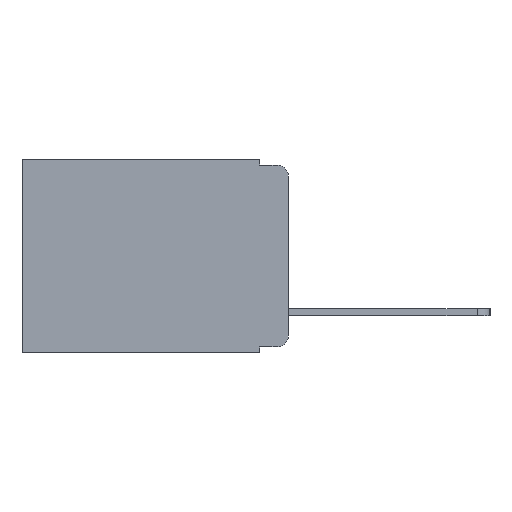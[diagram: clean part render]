
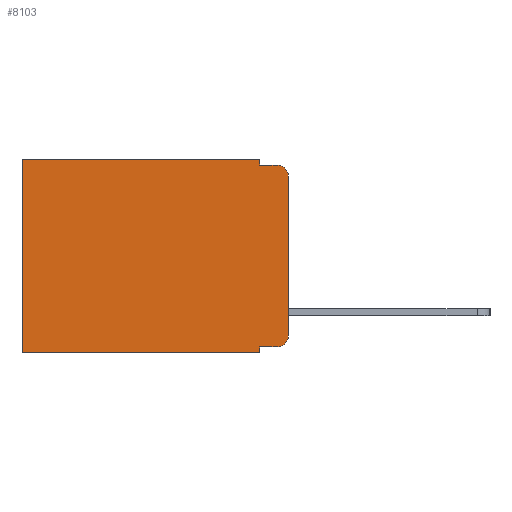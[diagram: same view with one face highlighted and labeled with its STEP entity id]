
A CAD part, left-side view. The second image highlights one B-rep face of the part: STEP entity #8103.
In plain terms, the highlighted planar face has unit normal (-1, 0, 0).
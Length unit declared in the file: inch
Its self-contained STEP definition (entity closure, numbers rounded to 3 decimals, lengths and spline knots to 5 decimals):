
#501 = EDGE_CURVE ( 'NONE', #8266, #10740, #7500, .T. ) ;
#517 = VECTOR ( 'NONE', #9543, 39.37008 ) ;
#1205 = CARTESIAN_POINT ( 'NONE',  ( 0.298, 0., -0.03 ) ) ;
#1229 = LINE ( 'NONE', #2038, #6552 ) ;
#1471 = CARTESIAN_POINT ( 'NONE',  ( 0.298, 0.051, -0.01 ) ) ;
#1753 = CARTESIAN_POINT ( 'NONE',  ( 0.298, 0., -0.313 ) ) ;
#1886 = AXIS2_PLACEMENT_3D ( 'NONE', #12120, #12117, #11517 ) ;
#1944 = EDGE_CURVE ( 'NONE', #9816, #8266, #6136, .T. ) ;
#2038 = CARTESIAN_POINT ( 'NONE',  ( 0.298, 0.473, 0. ) ) ;
#2200 = AXIS2_PLACEMENT_3D ( 'NONE', #4067, #11360, #5139 ) ;
#2552 = CARTESIAN_POINT ( 'NONE',  ( 0.298, 0., 0. ) ) ;
#2587 = ORIENTED_EDGE ( 'NONE', *, *, #13192, .T. ) ;
#2833 = EDGE_CURVE ( 'NONE', #11687, #9010, #9664, .T. ) ;
#2908 = CARTESIAN_POINT ( 'NONE',  ( 0.298, 0.051, 0. ) ) ;
#2997 = EDGE_CURVE ( 'NONE', #3891, #12537, #10493, .T. ) ;
#3063 = ORIENTED_EDGE ( 'NONE', *, *, #11954, .F. ) ;
#3673 = LINE ( 'NONE', #8259, #8922 ) ;
#3827 = ORIENTED_EDGE ( 'NONE', *, *, #2833, .F. ) ;
#3891 = VERTEX_POINT ( 'NONE', #8270 ) ;
#4067 = CARTESIAN_POINT ( 'NONE',  ( 0.298, 0.02, -0.313 ) ) ;
#4087 = VECTOR ( 'NONE', #10235, 39.37008 ) ;
#4259 = CARTESIAN_POINT ( 'NONE',  ( 0.298, 0.02, -0.01 ) ) ;
#4471 = VECTOR ( 'NONE', #4760, 39.37008 ) ;
#4632 = VECTOR ( 'NONE', #11917, 39.37008 ) ;
#4685 = DIRECTION ( 'NONE',  ( 0., 0., -1. ) ) ;
#4690 = ORIENTED_EDGE ( 'NONE', *, *, #12621, .T. ) ;
#4722 = CARTESIAN_POINT ( 'NONE',  ( 0.298, 0.051, -0.01 ) ) ;
#4760 = DIRECTION ( 'NONE',  ( 0., -1., 0. ) ) ;
#4903 = VECTOR ( 'NONE', #12375, 39.37008 ) ;
#5139 = DIRECTION ( 'NONE',  ( 0., 0., -1. ) ) ;
#5840 = VERTEX_POINT ( 'NONE', #1753 ) ;
#5953 = EDGE_CURVE ( 'NONE', #12736, #9010, #7217, .T. ) ;
#6136 = LINE ( 'NONE', #9500, #517 ) ;
#6187 = ORIENTED_EDGE ( 'NONE', *, *, #11328, .F. ) ;
#6552 = VECTOR ( 'NONE', #9326, 39.37008 ) ;
#6600 = DIRECTION ( 'NONE',  ( 0., -1., 0. ) ) ;
#6691 = EDGE_LOOP ( 'NONE', ( #3063, #11713, #3827, #6187, #9414, #4690, #7978, #11766, #10893, #2587 ) ) ;
#6932 = EDGE_CURVE ( 'NONE', #9816, #9827, #3673, .T. ) ;
#7217 = CIRCLE ( 'NONE', #1886, 0.02 ) ;
#7500 = LINE ( 'NONE', #10459, #13256 ) ;
#7978 = ORIENTED_EDGE ( 'NONE', *, *, #501, .F. ) ;
#8103 = ADVANCED_FACE ( 'NONE', ( #12605 ), #9861, .F. ) ;
#8230 = CARTESIAN_POINT ( 'NONE',  ( 0.298, 0.473, -0.343 ) ) ;
#8259 = CARTESIAN_POINT ( 'NONE',  ( 0.298, 0.051, -0.333 ) ) ;
#8266 = VERTEX_POINT ( 'NONE', #9091 ) ;
#8270 = CARTESIAN_POINT ( 'NONE',  ( 0.298, 0.051, 0. ) ) ;
#8785 = CARTESIAN_POINT ( 'NONE',  ( 0.298, 0.02, -0.333 ) ) ;
#8922 = VECTOR ( 'NONE', #6600, 39.37008 ) ;
#9010 = VERTEX_POINT ( 'NONE', #4259 ) ;
#9091 = CARTESIAN_POINT ( 'NONE',  ( 0.298, 0.051, -0.343 ) ) ;
#9188 = CARTESIAN_POINT ( 'NONE',  ( 0.298, 0.473, 0. ) ) ;
#9326 = DIRECTION ( 'NONE',  ( 0., 0., -1. ) ) ;
#9414 = ORIENTED_EDGE ( 'NONE', *, *, #2997, .T. ) ;
#9500 = CARTESIAN_POINT ( 'NONE',  ( 0.298, 0.051, 0. ) ) ;
#9543 = DIRECTION ( 'NONE',  ( 0., 0., -1. ) ) ;
#9664 = LINE ( 'NONE', #4722, #4471 ) ;
#9816 = VERTEX_POINT ( 'NONE', #11867 ) ;
#9827 = VERTEX_POINT ( 'NONE', #8785 ) ;
#9861 = PLANE ( 'NONE',  #9883 ) ;
#9883 = AXIS2_PLACEMENT_3D ( 'NONE', #2552, #10917, #4685 ) ;
#9952 = LINE ( 'NONE', #2908, #4087 ) ;
#10235 = DIRECTION ( 'NONE',  ( 0., 0., -1. ) ) ;
#10459 = CARTESIAN_POINT ( 'NONE',  ( 0.298, 0., -0.343 ) ) ;
#10493 = LINE ( 'NONE', #12842, #4632 ) ;
#10740 = VERTEX_POINT ( 'NONE', #8230 ) ;
#10893 = ORIENTED_EDGE ( 'NONE', *, *, #6932, .T. ) ;
#10917 = DIRECTION ( 'NONE',  ( 1., 0., 0. ) ) ;
#11024 = DIRECTION ( 'NONE',  ( 0., 1., 0. ) ) ;
#11328 = EDGE_CURVE ( 'NONE', #3891, #11687, #9952, .T. ) ;
#11342 = CARTESIAN_POINT ( 'NONE',  ( 0.298, 0., 0. ) ) ;
#11360 = DIRECTION ( 'NONE',  ( -1., 0., 0. ) ) ;
#11517 = DIRECTION ( 'NONE',  ( 0., 0., -1. ) ) ;
#11687 = VERTEX_POINT ( 'NONE', #1471 ) ;
#11713 = ORIENTED_EDGE ( 'NONE', *, *, #5953, .T. ) ;
#11766 = ORIENTED_EDGE ( 'NONE', *, *, #1944, .F. ) ;
#11867 = CARTESIAN_POINT ( 'NONE',  ( 0.298, 0.051, -0.333 ) ) ;
#11917 = DIRECTION ( 'NONE',  ( 0., 1., 0. ) ) ;
#11954 = EDGE_CURVE ( 'NONE', #12736, #5840, #12822, .T. ) ;
#12117 = DIRECTION ( 'NONE',  ( -1., 0., 0. ) ) ;
#12120 = CARTESIAN_POINT ( 'NONE',  ( 0.298, 0.02, -0.03 ) ) ;
#12375 = DIRECTION ( 'NONE',  ( 0., 0., -1. ) ) ;
#12537 = VERTEX_POINT ( 'NONE', #9188 ) ;
#12605 = FACE_OUTER_BOUND ( 'NONE', #6691, .T. ) ;
#12621 = EDGE_CURVE ( 'NONE', #12537, #10740, #1229, .T. ) ;
#12736 = VERTEX_POINT ( 'NONE', #1205 ) ;
#12822 = LINE ( 'NONE', #11342, #4903 ) ;
#12842 = CARTESIAN_POINT ( 'NONE',  ( 0.298, 0., 0. ) ) ;
#13110 = CIRCLE ( 'NONE', #2200, 0.02 ) ;
#13192 = EDGE_CURVE ( 'NONE', #9827, #5840, #13110, .T. ) ;
#13256 = VECTOR ( 'NONE', #11024, 39.37008 ) ;
